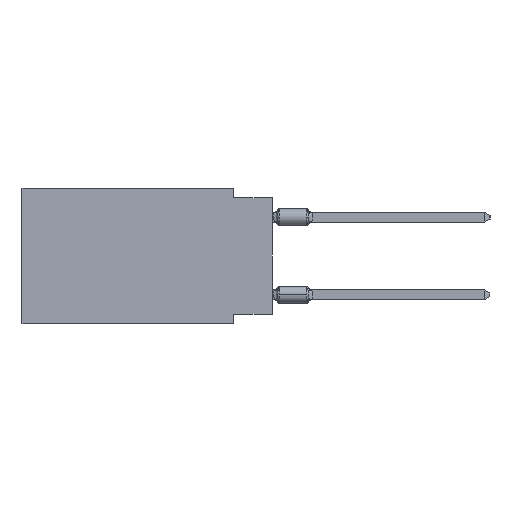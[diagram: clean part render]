
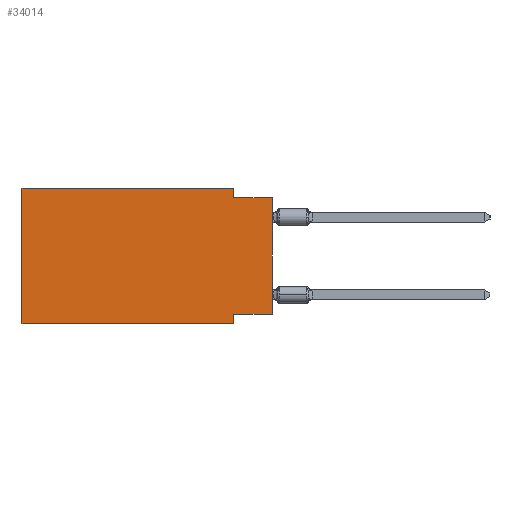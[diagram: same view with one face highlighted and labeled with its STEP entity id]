
A CAD part, left-side view. The second image highlights one B-rep face of the part: STEP entity #34014.
In plain terms, the highlighted planar face has unit normal (-1, 0, 0).
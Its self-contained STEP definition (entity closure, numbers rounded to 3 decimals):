
#1154 = LINE ( 'NONE', #9148, #27913 ) ;
#1773 = FACE_OUTER_BOUND ( 'NONE', #14464, .T. ) ;
#3862 = VECTOR ( 'NONE', #23001, 1000. ) ;
#4203 = DIRECTION ( 'NONE',  ( 0., 0., -1. ) ) ;
#4312 = CARTESIAN_POINT ( 'NONE',  ( 0., 16.383, 0. ) ) ;
#5858 = ORIENTED_EDGE ( 'NONE', *, *, #20327, .F. ) ;
#7197 = DIRECTION ( 'NONE',  ( 1., 0., 0. ) ) ;
#9148 = CARTESIAN_POINT ( 'NONE',  ( 0., 0., -8.255 ) ) ;
#9167 = VERTEX_POINT ( 'NONE', #26586 ) ;
#9337 = VERTEX_POINT ( 'NONE', #17337 ) ;
#9695 = VERTEX_POINT ( 'NONE', #23809 ) ;
#9804 = DIRECTION ( 'NONE',  ( 0., -1., 0. ) ) ;
#10029 = VECTOR ( 'NONE', #23765, 1000. ) ;
#10490 = CARTESIAN_POINT ( 'NONE',  ( 0., 2.54, -8.89 ) ) ;
#10766 = CARTESIAN_POINT ( 'NONE',  ( 0., 0., -0.635 ) ) ;
#11872 = DIRECTION ( 'NONE',  ( 0., 0., 1. ) ) ;
#11971 = EDGE_CURVE ( 'NONE', #26791, #33088, #17899, .T. ) ;
#12805 = ORIENTED_EDGE ( 'NONE', *, *, #20489, .F. ) ;
#12918 = LINE ( 'NONE', #10766, #10029 ) ;
#13453 = VECTOR ( 'NONE', #16765, 1000. ) ;
#13474 = ORIENTED_EDGE ( 'NONE', *, *, #16396, .F. ) ;
#13749 = ORIENTED_EDGE ( 'NONE', *, *, #30677, .T. ) ;
#14464 = EDGE_LOOP ( 'NONE', ( #24065, #12805, #13474, #32268, #18424, #13749, #15537, #5858 ) ) ;
#14691 = LINE ( 'NONE', #31495, #17161 ) ;
#14988 = AXIS2_PLACEMENT_3D ( 'NONE', #4312, #7197, #26395 ) ;
#15289 = DIRECTION ( 'NONE',  ( 0., 1., 0. ) ) ;
#15537 = ORIENTED_EDGE ( 'NONE', *, *, #18100, .F. ) ;
#15892 = VECTOR ( 'NONE', #20068, 1000. ) ;
#16396 = EDGE_CURVE ( 'NONE', #9167, #9695, #17938, .T. ) ;
#16437 = VECTOR ( 'NONE', #4203, 1000. ) ;
#16765 = DIRECTION ( 'NONE',  ( 0., -1., 0. ) ) ;
#17161 = VECTOR ( 'NONE', #9804, 1000. ) ;
#17337 = CARTESIAN_POINT ( 'NONE',  ( 0., 16.383, 0. ) ) ;
#17899 = LINE ( 'NONE', #22964, #15892 ) ;
#17938 = LINE ( 'NONE', #18113, #3862 ) ;
#18100 = EDGE_CURVE ( 'NONE', #26390, #24703, #18328, .T. ) ;
#18113 = CARTESIAN_POINT ( 'NONE',  ( 0., 2.54, 0. ) ) ;
#18328 = LINE ( 'NONE', #23193, #16437 ) ;
#18424 = ORIENTED_EDGE ( 'NONE', *, *, #19428, .F. ) ;
#19246 = VERTEX_POINT ( 'NONE', #35556 ) ;
#19428 = EDGE_CURVE ( 'NONE', #19246, #9337, #31208, .T. ) ;
#20068 = DIRECTION ( 'NONE',  ( 0., 0., 1. ) ) ;
#20197 = EDGE_CURVE ( 'NONE', #9337, #9167, #33190, .T. ) ;
#20327 = EDGE_CURVE ( 'NONE', #26791, #26390, #1154, .T. ) ;
#20489 = EDGE_CURVE ( 'NONE', #9695, #33088, #12918, .T. ) ;
#21498 = VECTOR ( 'NONE', #11872, 1000. ) ;
#22247 = CARTESIAN_POINT ( 'NONE',  ( 0., 0., -8.255 ) ) ;
#22696 = CARTESIAN_POINT ( 'NONE',  ( 0., 16.383, 0. ) ) ;
#22964 = CARTESIAN_POINT ( 'NONE',  ( 0., 0., 0. ) ) ;
#23001 = DIRECTION ( 'NONE',  ( 0., 0., -1. ) ) ;
#23193 = CARTESIAN_POINT ( 'NONE',  ( 0., 2.54, -8.89 ) ) ;
#23765 = DIRECTION ( 'NONE',  ( 0., -1., 0. ) ) ;
#23809 = CARTESIAN_POINT ( 'NONE',  ( 0., 2.54, -0.635 ) ) ;
#24065 = ORIENTED_EDGE ( 'NONE', *, *, #11971, .T. ) ;
#24703 = VERTEX_POINT ( 'NONE', #10490 ) ;
#26141 = CARTESIAN_POINT ( 'NONE',  ( 0., 16.383, 0. ) ) ;
#26390 = VERTEX_POINT ( 'NONE', #33477 ) ;
#26395 = DIRECTION ( 'NONE',  ( 0., 0., -1. ) ) ;
#26586 = CARTESIAN_POINT ( 'NONE',  ( 0., 2.54, 0. ) ) ;
#26791 = VERTEX_POINT ( 'NONE', #22247 ) ;
#27913 = VECTOR ( 'NONE', #15289, 1000. ) ;
#29089 = PLANE ( 'NONE',  #14988 ) ;
#30677 = EDGE_CURVE ( 'NONE', #19246, #24703, #14691, .T. ) ;
#31208 = LINE ( 'NONE', #26141, #21498 ) ;
#31495 = CARTESIAN_POINT ( 'NONE',  ( 0., 16.383, -8.89 ) ) ;
#31873 = CARTESIAN_POINT ( 'NONE',  ( 0., 0., -0.635 ) ) ;
#32268 = ORIENTED_EDGE ( 'NONE', *, *, #20197, .F. ) ;
#33088 = VERTEX_POINT ( 'NONE', #31873 ) ;
#33190 = LINE ( 'NONE', #22696, #13453 ) ;
#33477 = CARTESIAN_POINT ( 'NONE',  ( 0., 2.54, -8.255 ) ) ;
#34014 = ADVANCED_FACE ( 'NONE', ( #1773 ), #29089, .F. ) ;
#35556 = CARTESIAN_POINT ( 'NONE',  ( 0., 16.383, -8.89 ) ) ;
